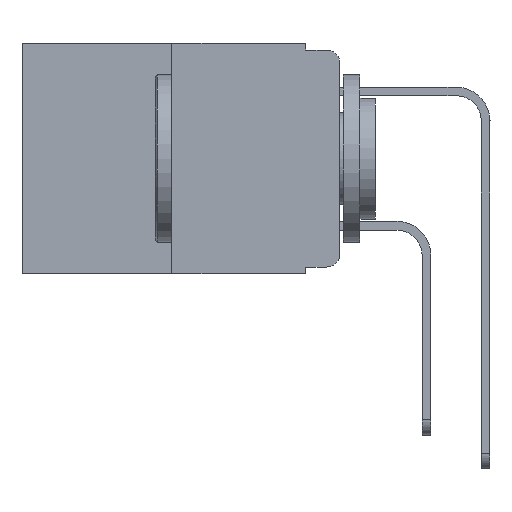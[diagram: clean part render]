
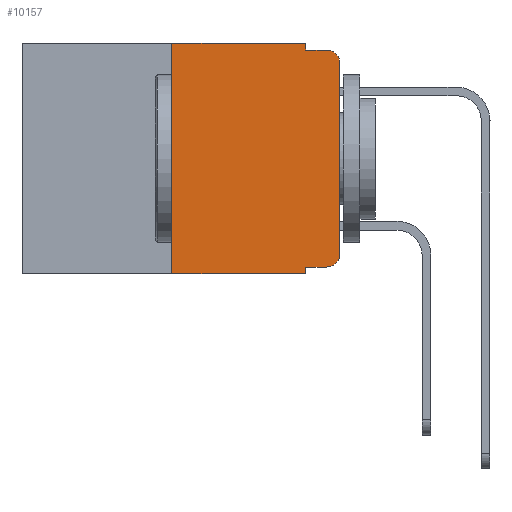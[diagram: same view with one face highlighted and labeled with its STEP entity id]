
A CAD part, left-side view. The second image highlights one B-rep face of the part: STEP entity #10157.
In plain terms, the highlighted planar face has unit normal (-1, 0, 0).
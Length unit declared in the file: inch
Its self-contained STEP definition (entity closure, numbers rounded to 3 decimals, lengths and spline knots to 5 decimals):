
#45 = DIRECTION ( 'NONE',  ( -1., 0., 0. ) ) ;
#198 = ORIENTED_EDGE ( 'NONE', *, *, #667, .T. ) ;
#667 = EDGE_CURVE ( 'NONE', #16504, #11066, #10201, .T. ) ;
#1965 = ORIENTED_EDGE ( 'NONE', *, *, #5419, .F. ) ;
#2017 = CARTESIAN_POINT ( 'NONE',  ( 0., 0., -0.03 ) ) ;
#2152 = DIRECTION ( 'NONE',  ( 0., -1., 0. ) ) ;
#2176 = EDGE_CURVE ( 'NONE', #16504, #21158, #24771, .T. ) ;
#2429 = LINE ( 'NONE', #26847, #24776 ) ;
#2513 = DIRECTION ( 'NONE',  ( 0., 0., -1. ) ) ;
#3650 = AXIS2_PLACEMENT_3D ( 'NONE', #21762, #8962, #23844 ) ;
#4896 = VECTOR ( 'NONE', #27894, 39.37008 ) ;
#5419 = EDGE_CURVE ( 'NONE', #12638, #9898, #16063, .T. ) ;
#5841 = ORIENTED_EDGE ( 'NONE', *, *, #16927, .T. ) ;
#6521 = VERTEX_POINT ( 'NONE', #12489 ) ;
#6716 = EDGE_CURVE ( 'NONE', #25044, #12638, #12044, .T. ) ;
#6732 = CARTESIAN_POINT ( 'NONE',  ( 0., 0.051, 0. ) ) ;
#6918 = ORIENTED_EDGE ( 'NONE', *, *, #27257, .T. ) ;
#7771 = VECTOR ( 'NONE', #2513, 39.37008 ) ;
#8258 = EDGE_CURVE ( 'NONE', #9898, #17018, #24433, .T. ) ;
#8598 = EDGE_LOOP ( 'NONE', ( #11078, #5841, #23039, #18145, #1965, #15144, #21400, #11434, #198, #6918 ) ) ;
#8807 = DIRECTION ( 'NONE',  ( 0., 0., 1. ) ) ;
#8946 = DIRECTION ( 'NONE',  ( 1., 0., 0. ) ) ;
#8962 = DIRECTION ( 'NONE',  ( -1., 0., 0. ) ) ;
#9315 = CARTESIAN_POINT ( 'NONE',  ( 0., 0.051, -0.01 ) ) ;
#9417 = CIRCLE ( 'NONE', #13517, 0.02 ) ;
#9898 = VERTEX_POINT ( 'NONE', #14486 ) ;
#10070 = CARTESIAN_POINT ( 'NONE',  ( 0., 0.02, -0.01 ) ) ;
#10157 = ADVANCED_FACE ( 'NONE', ( #18822 ), #25816, .F. ) ;
#10201 = LINE ( 'NONE', #26421, #4896 ) ;
#10340 = VECTOR ( 'NONE', #12886, 39.37008 ) ;
#10936 = LINE ( 'NONE', #21308, #21591 ) ;
#11066 = VERTEX_POINT ( 'NONE', #25938 ) ;
#11078 = ORIENTED_EDGE ( 'NONE', *, *, #19783, .T. ) ;
#11434 = ORIENTED_EDGE ( 'NONE', *, *, #2176, .F. ) ;
#12044 = LINE ( 'NONE', #25775, #22610 ) ;
#12289 = VECTOR ( 'NONE', #2152, 39.37008 ) ;
#12391 = CARTESIAN_POINT ( 'NONE',  ( 0., 0.25, 0. ) ) ;
#12489 = CARTESIAN_POINT ( 'NONE',  ( 0., 0., -0.313 ) ) ;
#12638 = VERTEX_POINT ( 'NONE', #12391 ) ;
#12886 = DIRECTION ( 'NONE',  ( 0., -1., 0. ) ) ;
#13422 = CARTESIAN_POINT ( 'NONE',  ( 0., 0.02, -0.03 ) ) ;
#13517 = AXIS2_PLACEMENT_3D ( 'NONE', #13422, #45, #15577 ) ;
#13521 = DIRECTION ( 'NONE',  ( 0., 0., -1. ) ) ;
#14486 = CARTESIAN_POINT ( 'NONE',  ( 0., 0.051, 0. ) ) ;
#15144 = ORIENTED_EDGE ( 'NONE', *, *, #6716, .F. ) ;
#15540 = EDGE_CURVE ( 'NONE', #17018, #19611, #23482, .T. ) ;
#15577 = DIRECTION ( 'NONE',  ( 0., 0., -1. ) ) ;
#15892 = EDGE_CURVE ( 'NONE', #25044, #21158, #2429, .T. ) ;
#16063 = LINE ( 'NONE', #19211, #10340 ) ;
#16504 = VERTEX_POINT ( 'NONE', #20552 ) ;
#16927 = EDGE_CURVE ( 'NONE', #27834, #19611, #9417, .T. ) ;
#17018 = VERTEX_POINT ( 'NONE', #9315 ) ;
#18145 = ORIENTED_EDGE ( 'NONE', *, *, #8258, .F. ) ;
#18822 = FACE_OUTER_BOUND ( 'NONE', #8598, .T. ) ;
#19211 = CARTESIAN_POINT ( 'NONE',  ( 0., 0.473, 0. ) ) ;
#19560 = VECTOR ( 'NONE', #13521, 39.37008 ) ;
#19611 = VERTEX_POINT ( 'NONE', #10070 ) ;
#19783 = EDGE_CURVE ( 'NONE', #6521, #27834, #10936, .T. ) ;
#20552 = CARTESIAN_POINT ( 'NONE',  ( 0., 0.051, -0.333 ) ) ;
#21158 = VERTEX_POINT ( 'NONE', #23606 ) ;
#21308 = CARTESIAN_POINT ( 'NONE',  ( 0., 0., 0. ) ) ;
#21400 = ORIENTED_EDGE ( 'NONE', *, *, #15892, .T. ) ;
#21591 = VECTOR ( 'NONE', #23402, 39.37008 ) ;
#21738 = CARTESIAN_POINT ( 'NONE',  ( 0., 0.473, 0. ) ) ;
#21762 = CARTESIAN_POINT ( 'NONE',  ( 0., 0.02, -0.313 ) ) ;
#22610 = VECTOR ( 'NONE', #8807, 39.37008 ) ;
#23039 = ORIENTED_EDGE ( 'NONE', *, *, #15540, .F. ) ;
#23402 = DIRECTION ( 'NONE',  ( 0., 0., 1. ) ) ;
#23482 = LINE ( 'NONE', #27918, #12289 ) ;
#23606 = CARTESIAN_POINT ( 'NONE',  ( 0., 0.051, -0.343 ) ) ;
#23787 = AXIS2_PLACEMENT_3D ( 'NONE', #21738, #8946, #23825 ) ;
#23825 = DIRECTION ( 'NONE',  ( 0., 0., -1. ) ) ;
#23844 = DIRECTION ( 'NONE',  ( 0., 0., -1. ) ) ;
#24433 = LINE ( 'NONE', #26083, #19560 ) ;
#24468 = CARTESIAN_POINT ( 'NONE',  ( 0., 0.25, -0.343 ) ) ;
#24771 = LINE ( 'NONE', #6732, #7771 ) ;
#24776 = VECTOR ( 'NONE', #24841, 39.37008 ) ;
#24841 = DIRECTION ( 'NONE',  ( 0., -1., 0. ) ) ;
#25044 = VERTEX_POINT ( 'NONE', #24468 ) ;
#25099 = CIRCLE ( 'NONE', #3650, 0.02 ) ;
#25775 = CARTESIAN_POINT ( 'NONE',  ( 0., 0.25, 0. ) ) ;
#25816 = PLANE ( 'NONE',  #23787 ) ;
#25938 = CARTESIAN_POINT ( 'NONE',  ( 0., 0.02, -0.333 ) ) ;
#26083 = CARTESIAN_POINT ( 'NONE',  ( 0., 0.051, 0. ) ) ;
#26421 = CARTESIAN_POINT ( 'NONE',  ( 0., 0.051, -0.333 ) ) ;
#26847 = CARTESIAN_POINT ( 'NONE',  ( 0., 0.473, -0.343 ) ) ;
#27257 = EDGE_CURVE ( 'NONE', #11066, #6521, #25099, .T. ) ;
#27834 = VERTEX_POINT ( 'NONE', #2017 ) ;
#27894 = DIRECTION ( 'NONE',  ( 0., -1., 0. ) ) ;
#27918 = CARTESIAN_POINT ( 'NONE',  ( 0., 0.051, -0.01 ) ) ;
